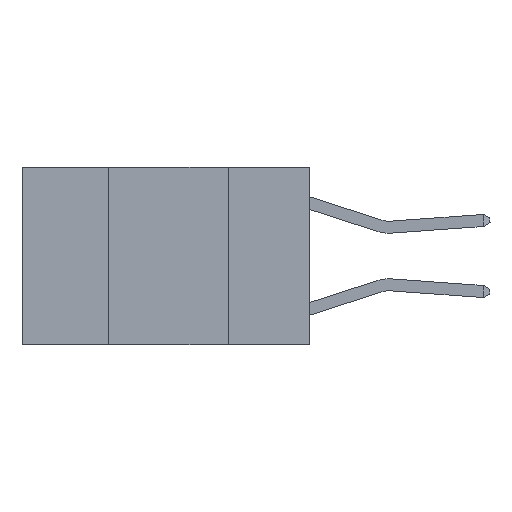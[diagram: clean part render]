
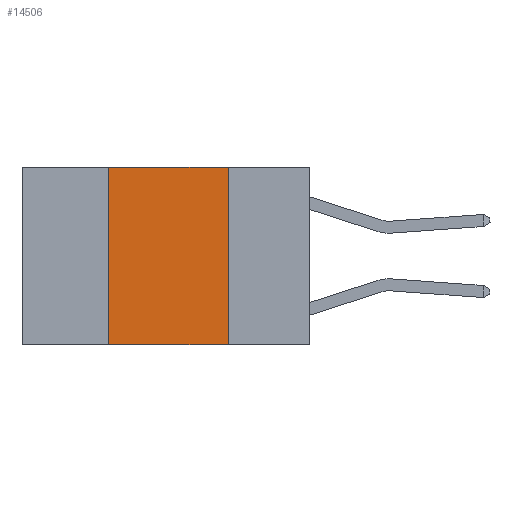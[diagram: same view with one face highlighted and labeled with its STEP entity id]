
A CAD part, left-side view. The second image highlights one B-rep face of the part: STEP entity #14506.
In plain terms, the highlighted planar face has unit normal (-1, 0, 0).
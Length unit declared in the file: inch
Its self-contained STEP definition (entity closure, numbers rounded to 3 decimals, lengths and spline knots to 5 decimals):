
#50 = LINE ( 'NONE', #10955, #3069 ) ;
#214 = CARTESIAN_POINT ( 'NONE',  ( 0., 0.6, 0. ) ) ;
#401 = CARTESIAN_POINT ( 'NONE',  ( 0., 0.17, 0. ) ) ;
#910 = ORIENTED_EDGE ( 'NONE', *, *, #3349, .F. ) ;
#933 = LINE ( 'NONE', #3471, #7415 ) ;
#1060 = EDGE_CURVE ( 'NONE', #4068, #13507, #50, .T. ) ;
#1097 = CARTESIAN_POINT ( 'NONE',  ( 0., 0.17, 0. ) ) ;
#1490 = VERTEX_POINT ( 'NONE', #401 ) ;
#1671 = EDGE_CURVE ( 'NONE', #1490, #13507, #5890, .T. ) ;
#2143 = DIRECTION ( 'NONE',  ( 0., 0., 1. ) ) ;
#2428 = CARTESIAN_POINT ( 'NONE',  ( 0., 0.42, 0. ) ) ;
#2708 = ORIENTED_EDGE ( 'NONE', *, *, #1060, .T. ) ;
#3069 = VECTOR ( 'NONE', #14449, 39.37008 ) ;
#3349 = EDGE_CURVE ( 'NONE', #4068, #12755, #3642, .T. ) ;
#3471 = CARTESIAN_POINT ( 'NONE',  ( 0., 0.6, 0. ) ) ;
#3642 = LINE ( 'NONE', #2428, #5857 ) ;
#4068 = VERTEX_POINT ( 'NONE', #14517 ) ;
#4113 = DIRECTION ( 'NONE',  ( 0., 0., -1. ) ) ;
#4723 = CARTESIAN_POINT ( 'NONE',  ( 0., 0.17, -0.37 ) ) ;
#5857 = VECTOR ( 'NONE', #2143, 39.37008 ) ;
#5890 = LINE ( 'NONE', #1097, #15817 ) ;
#7257 = ORIENTED_EDGE ( 'NONE', *, *, #11704, .F. ) ;
#7415 = VECTOR ( 'NONE', #13853, 39.37008 ) ;
#7714 = EDGE_LOOP ( 'NONE', ( #14077, #7257, #910, #2708 ) ) ;
#8153 = FACE_OUTER_BOUND ( 'NONE', #7714, .T. ) ;
#9618 = CARTESIAN_POINT ( 'NONE',  ( 0., 0.42, 0. ) ) ;
#9997 = AXIS2_PLACEMENT_3D ( 'NONE', #214, #11872, #4113 ) ;
#10955 = CARTESIAN_POINT ( 'NONE',  ( 0., 0.6, -0.37 ) ) ;
#11704 = EDGE_CURVE ( 'NONE', #12755, #1490, #933, .T. ) ;
#11872 = DIRECTION ( 'NONE',  ( 1., 0., 0. ) ) ;
#12755 = VERTEX_POINT ( 'NONE', #9618 ) ;
#13507 = VERTEX_POINT ( 'NONE', #4723 ) ;
#13853 = DIRECTION ( 'NONE',  ( 0., -1., 0. ) ) ;
#14002 = DIRECTION ( 'NONE',  ( 0., 0., -1. ) ) ;
#14077 = ORIENTED_EDGE ( 'NONE', *, *, #1671, .F. ) ;
#14425 = PLANE ( 'NONE',  #9997 ) ;
#14449 = DIRECTION ( 'NONE',  ( 0., -1., 0. ) ) ;
#14506 = ADVANCED_FACE ( 'NONE', ( #8153 ), #14425, .F. ) ;
#14517 = CARTESIAN_POINT ( 'NONE',  ( 0., 0.42, -0.37 ) ) ;
#15817 = VECTOR ( 'NONE', #14002, 39.37008 ) ;
